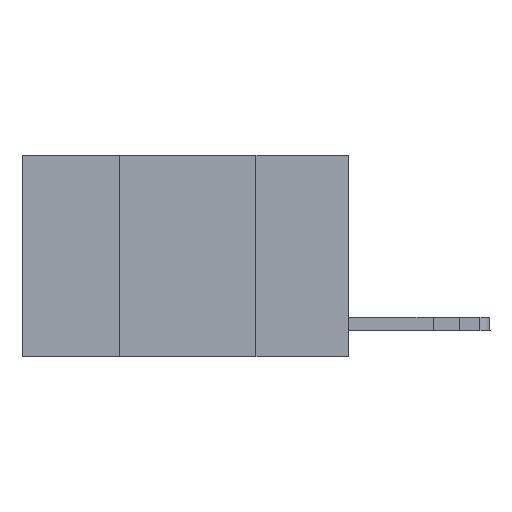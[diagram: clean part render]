
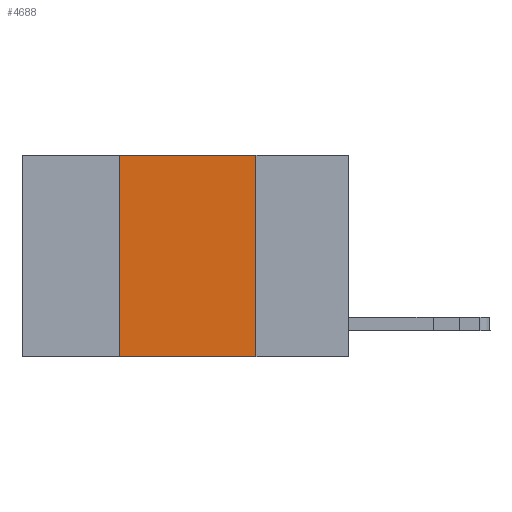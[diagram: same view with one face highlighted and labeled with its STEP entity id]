
A CAD part, left-side view. The second image highlights one B-rep face of the part: STEP entity #4688.
In plain terms, the highlighted planar face has unit normal (-1, 0, 0).
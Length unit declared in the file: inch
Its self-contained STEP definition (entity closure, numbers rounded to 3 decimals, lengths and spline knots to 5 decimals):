
#220 = CARTESIAN_POINT ( 'NONE',  ( 0., 0.42, 0. ) ) ;
#249 = AXIS2_PLACEMENT_3D ( 'NONE', #1769, #3807, #10198 ) ;
#782 = PLANE ( 'NONE',  #249 ) ;
#935 = VECTOR ( 'NONE', #11647, 39.37008 ) ;
#1326 = DIRECTION ( 'NONE',  ( 0., 0., -1. ) ) ;
#1380 = EDGE_CURVE ( 'NONE', #5970, #4109, #8269, .T. ) ;
#1408 = VERTEX_POINT ( 'NONE', #1708 ) ;
#1411 = CARTESIAN_POINT ( 'NONE',  ( 0., 0.42, 0. ) ) ;
#1708 = CARTESIAN_POINT ( 'NONE',  ( 0., 0.17, 0. ) ) ;
#1769 = CARTESIAN_POINT ( 'NONE',  ( 0., 0.6, 0. ) ) ;
#3807 = DIRECTION ( 'NONE',  ( 1., 0., 0. ) ) ;
#3913 = DIRECTION ( 'NONE',  ( 0., -1., 0. ) ) ;
#4109 = VERTEX_POINT ( 'NONE', #220 ) ;
#4291 = EDGE_CURVE ( 'NONE', #5970, #8938, #9250, .T. ) ;
#4688 = ADVANCED_FACE ( 'NONE', ( #9375 ), #782, .F. ) ;
#4929 = EDGE_CURVE ( 'NONE', #4109, #1408, #7575, .T. ) ;
#4938 = EDGE_CURVE ( 'NONE', #1408, #8938, #11682, .T. ) ;
#5180 = ORIENTED_EDGE ( 'NONE', *, *, #1380, .F. ) ;
#5970 = VERTEX_POINT ( 'NONE', #7425 ) ;
#6380 = EDGE_LOOP ( 'NONE', ( #8990, #10513, #5180, #10181 ) ) ;
#7425 = CARTESIAN_POINT ( 'NONE',  ( 0., 0.42, -0.37 ) ) ;
#7464 = VECTOR ( 'NONE', #3913, 39.37008 ) ;
#7575 = LINE ( 'NONE', #11481, #9635 ) ;
#7986 = DIRECTION ( 'NONE',  ( 0., -1., 0. ) ) ;
#8269 = LINE ( 'NONE', #1411, #935 ) ;
#8938 = VERTEX_POINT ( 'NONE', #11379 ) ;
#8990 = ORIENTED_EDGE ( 'NONE', *, *, #4938, .F. ) ;
#9250 = LINE ( 'NONE', #9398, #7464 ) ;
#9367 = VECTOR ( 'NONE', #1326, 39.37008 ) ;
#9375 = FACE_OUTER_BOUND ( 'NONE', #6380, .T. ) ;
#9398 = CARTESIAN_POINT ( 'NONE',  ( 0., 0.6, -0.37 ) ) ;
#9635 = VECTOR ( 'NONE', #7986, 39.37008 ) ;
#10181 = ORIENTED_EDGE ( 'NONE', *, *, #4291, .T. ) ;
#10198 = DIRECTION ( 'NONE',  ( 0., 0., -1. ) ) ;
#10513 = ORIENTED_EDGE ( 'NONE', *, *, #4929, .F. ) ;
#11379 = CARTESIAN_POINT ( 'NONE',  ( 0., 0.17, -0.37 ) ) ;
#11481 = CARTESIAN_POINT ( 'NONE',  ( 0., 0.6, 0. ) ) ;
#11517 = CARTESIAN_POINT ( 'NONE',  ( 0., 0.17, 0. ) ) ;
#11647 = DIRECTION ( 'NONE',  ( 0., 0., 1. ) ) ;
#11682 = LINE ( 'NONE', #11517, #9367 ) ;
